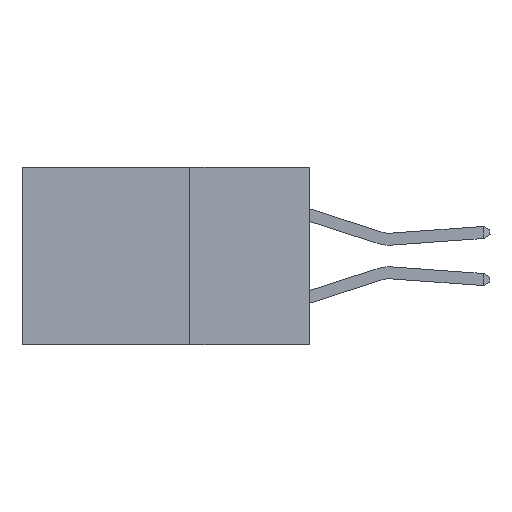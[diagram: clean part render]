
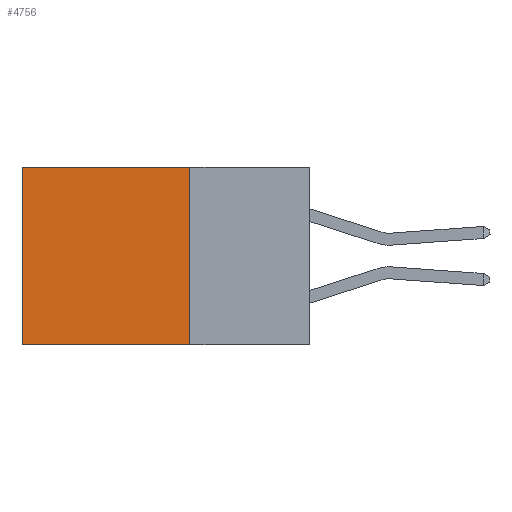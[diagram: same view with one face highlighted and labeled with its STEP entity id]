
A CAD part, left-side view. The second image highlights one B-rep face of the part: STEP entity #4756.
In plain terms, the highlighted planar face has unit normal (-1, 0, 0).
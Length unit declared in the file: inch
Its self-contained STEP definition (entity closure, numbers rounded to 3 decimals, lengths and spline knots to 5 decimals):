
#611 = VECTOR ( 'NONE', #9966, 39.37008 ) ;
#905 = CARTESIAN_POINT ( 'NONE',  ( 0.2615, 0.25, 0. ) ) ;
#1326 = EDGE_CURVE ( 'NONE', #1873, #7706, #14523, .T. ) ;
#1572 = LINE ( 'NONE', #13497, #611 ) ;
#1804 = LINE ( 'NONE', #7393, #5842 ) ;
#1873 = VERTEX_POINT ( 'NONE', #905 ) ;
#2555 = CARTESIAN_POINT ( 'NONE',  ( 0.2615, 0.25, -0.37 ) ) ;
#2668 = EDGE_CURVE ( 'NONE', #10506, #11151, #1804, .T. ) ;
#3869 = DIRECTION ( 'NONE',  ( 1., 0., 0. ) ) ;
#4317 = DIRECTION ( 'NONE',  ( 0., 0., -1. ) ) ;
#4504 = EDGE_LOOP ( 'NONE', ( #11246, #10905, #8056, #14903 ) ) ;
#4756 = ADVANCED_FACE ( 'NONE', ( #8454 ), #13159, .F. ) ;
#5210 = CARTESIAN_POINT ( 'NONE',  ( 0.2615, 0.25, -0.37 ) ) ;
#5842 = VECTOR ( 'NONE', #13358, 39.37008 ) ;
#6063 = DIRECTION ( 'NONE',  ( 0., 1., 0. ) ) ;
#6791 = VECTOR ( 'NONE', #6063, 39.37008 ) ;
#7393 = CARTESIAN_POINT ( 'NONE',  ( 0.2615, 0.25, -0.37 ) ) ;
#7559 = EDGE_CURVE ( 'NONE', #1873, #10506, #1572, .T. ) ;
#7671 = AXIS2_PLACEMENT_3D ( 'NONE', #2555, #3869, #9860 ) ;
#7706 = VERTEX_POINT ( 'NONE', #11422 ) ;
#8056 = ORIENTED_EDGE ( 'NONE', *, *, #7559, .F. ) ;
#8454 = FACE_OUTER_BOUND ( 'NONE', #4504, .T. ) ;
#8859 = CARTESIAN_POINT ( 'NONE',  ( 0.2615, 0.25, 0. ) ) ;
#9860 = DIRECTION ( 'NONE',  ( 0., 0., -1. ) ) ;
#9966 = DIRECTION ( 'NONE',  ( 0., 0., -1. ) ) ;
#10154 = LINE ( 'NONE', #14851, #12501 ) ;
#10506 = VERTEX_POINT ( 'NONE', #5210 ) ;
#10905 = ORIENTED_EDGE ( 'NONE', *, *, #2668, .F. ) ;
#11035 = EDGE_CURVE ( 'NONE', #7706, #11151, #10154, .T. ) ;
#11151 = VERTEX_POINT ( 'NONE', #13917 ) ;
#11246 = ORIENTED_EDGE ( 'NONE', *, *, #11035, .T. ) ;
#11422 = CARTESIAN_POINT ( 'NONE',  ( 0.2615, 0.6, 0. ) ) ;
#12501 = VECTOR ( 'NONE', #4317, 39.37008 ) ;
#13159 = PLANE ( 'NONE',  #7671 ) ;
#13358 = DIRECTION ( 'NONE',  ( 0., 1., 0. ) ) ;
#13497 = CARTESIAN_POINT ( 'NONE',  ( 0.2615, 0.25, -0.37 ) ) ;
#13917 = CARTESIAN_POINT ( 'NONE',  ( 0.2615, 0.6, -0.37 ) ) ;
#14523 = LINE ( 'NONE', #8859, #6791 ) ;
#14851 = CARTESIAN_POINT ( 'NONE',  ( 0.2615, 0.6, -0.37 ) ) ;
#14903 = ORIENTED_EDGE ( 'NONE', *, *, #1326, .T. ) ;
